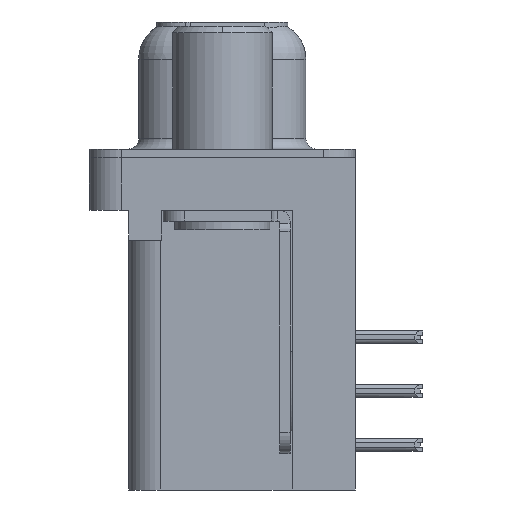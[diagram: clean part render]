
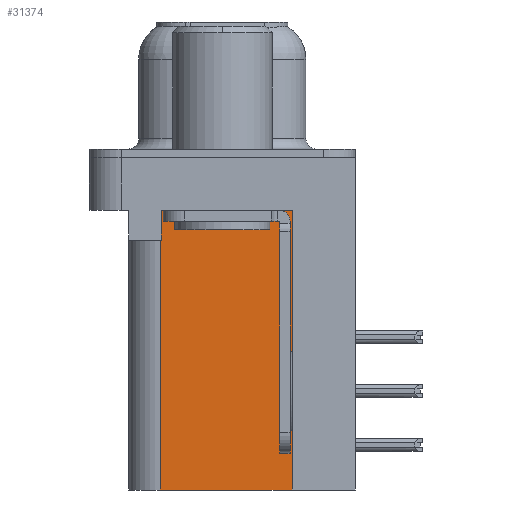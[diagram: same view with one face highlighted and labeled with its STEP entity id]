
A CAD part, left-side view. The second image highlights one B-rep face of the part: STEP entity #31374.
In plain terms, the highlighted planar face has unit normal (-1, 0, 0).
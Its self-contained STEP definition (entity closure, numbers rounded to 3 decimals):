
#3 = EDGE_CURVE ( 'NONE', #13796, #28447, #30873, .T. ) ;
#520 = DIRECTION ( 'NONE',  ( 0., 1., 0. ) ) ;
#1145 = DIRECTION ( 'NONE',  ( 0., 1., 0. ) ) ;
#1280 = ORIENTED_EDGE ( 'NONE', *, *, #7685, .T. ) ;
#1394 = EDGE_CURVE ( 'NONE', #29479, #6964, #3757, .T. ) ;
#2110 = CARTESIAN_POINT ( 'NONE',  ( 3.765, 2.925, -15.7 ) ) ;
#3571 = EDGE_CURVE ( 'NONE', #7024, #13796, #24205, .T. ) ;
#3757 = LINE ( 'NONE', #37428, #18693 ) ;
#4413 = CARTESIAN_POINT ( 'NONE',  ( 3.765, 2.925, -3.9 ) ) ;
#6964 = VERTEX_POINT ( 'NONE', #21142 ) ;
#7024 = VERTEX_POINT ( 'NONE', #33214 ) ;
#7685 = EDGE_CURVE ( 'NONE', #19701, #28447, #28221, .T. ) ;
#7749 = CARTESIAN_POINT ( 'NONE',  ( 3.765, -3.295, -15.7 ) ) ;
#7855 = CARTESIAN_POINT ( 'NONE',  ( 3.765, 2.895, -3.9 ) ) ;
#9865 = CARTESIAN_POINT ( 'NONE',  ( 3.765, 0., -3.9 ) ) ;
#9941 = ORIENTED_EDGE ( 'NONE', *, *, #29168, .T. ) ;
#13057 = PLANE ( 'NONE',  #36607 ) ;
#13508 = EDGE_CURVE ( 'NONE', #6964, #19701, #21258, .T. ) ;
#13796 = VERTEX_POINT ( 'NONE', #2110 ) ;
#15289 = VECTOR ( 'NONE', #520, 1000. ) ;
#16041 = CARTESIAN_POINT ( 'NONE',  ( 3.765, -3.295, -15.7 ) ) ;
#16839 = LINE ( 'NONE', #7749, #23899 ) ;
#18693 = VECTOR ( 'NONE', #19337, 1000. ) ;
#19045 = DIRECTION ( 'NONE',  ( 1., 0., 0. ) ) ;
#19212 = DIRECTION ( 'NONE',  ( 0., 0., 1. ) ) ;
#19335 = CARTESIAN_POINT ( 'NONE',  ( 3.765, 2.925, -15.7 ) ) ;
#19337 = DIRECTION ( 'NONE',  ( 0., 1., 0. ) ) ;
#19701 = VERTEX_POINT ( 'NONE', #7855 ) ;
#20744 = ORIENTED_EDGE ( 'NONE', *, *, #13508, .T. ) ;
#20788 = EDGE_LOOP ( 'NONE', ( #21456, #20744, #1280, #38699, #21923, #9941 ) ) ;
#21142 = CARTESIAN_POINT ( 'NONE',  ( 3.765, 2.895, -2.5 ) ) ;
#21210 = VECTOR ( 'NONE', #33816, 1000. ) ;
#21258 = LINE ( 'NONE', #29920, #35304 ) ;
#21456 = ORIENTED_EDGE ( 'NONE', *, *, #1394, .T. ) ;
#21923 = ORIENTED_EDGE ( 'NONE', *, *, #3571, .F. ) ;
#22782 = DIRECTION ( 'NONE',  ( 0., 0., 1. ) ) ;
#22826 = VECTOR ( 'NONE', #19212, 1000. ) ;
#23899 = VECTOR ( 'NONE', #22782, 1000. ) ;
#24205 = LINE ( 'NONE', #24454, #15289 ) ;
#24454 = CARTESIAN_POINT ( 'NONE',  ( 3.765, -3.295, -15.7 ) ) ;
#24628 = CARTESIAN_POINT ( 'NONE',  ( 3.765, -3.295, -2.5 ) ) ;
#27525 = FACE_OUTER_BOUND ( 'NONE', #20788, .T. ) ;
#28221 = LINE ( 'NONE', #9865, #21210 ) ;
#28447 = VERTEX_POINT ( 'NONE', #4413 ) ;
#29168 = EDGE_CURVE ( 'NONE', #7024, #29479, #16839, .T. ) ;
#29479 = VERTEX_POINT ( 'NONE', #24628 ) ;
#29920 = CARTESIAN_POINT ( 'NONE',  ( 3.765, 2.895, -3.9 ) ) ;
#30873 = LINE ( 'NONE', #19335, #22826 ) ;
#31374 = ADVANCED_FACE ( 'NONE', ( #27525 ), #13057, .F. ) ;
#32930 = DIRECTION ( 'NONE',  ( 0., 0., -1. ) ) ;
#33214 = CARTESIAN_POINT ( 'NONE',  ( 3.765, -3.295, -15.7 ) ) ;
#33816 = DIRECTION ( 'NONE',  ( 0., 1., 0. ) ) ;
#35304 = VECTOR ( 'NONE', #32930, 1000. ) ;
#36607 = AXIS2_PLACEMENT_3D ( 'NONE', #16041, #19045, #1145 ) ;
#37428 = CARTESIAN_POINT ( 'NONE',  ( 3.765, -3.295, -2.5 ) ) ;
#38699 = ORIENTED_EDGE ( 'NONE', *, *, #3, .F. ) ;
